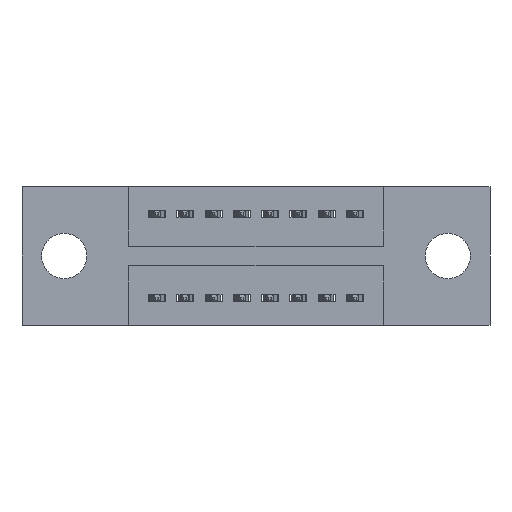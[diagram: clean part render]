
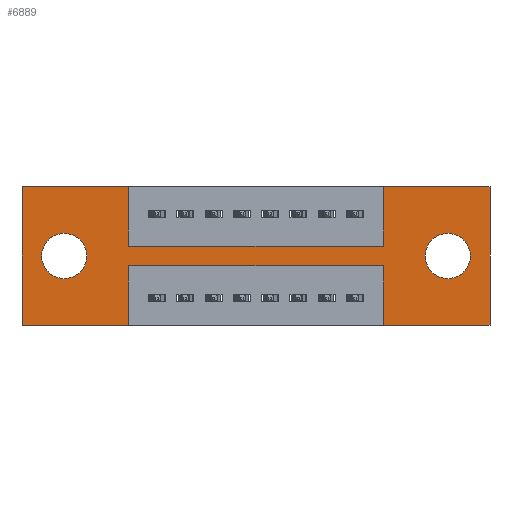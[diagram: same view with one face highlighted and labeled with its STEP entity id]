
A CAD part, front view. The second image highlights one B-rep face of the part: STEP entity #6889.
In plain terms, the highlighted planar face has unit normal (0, -1, 0).
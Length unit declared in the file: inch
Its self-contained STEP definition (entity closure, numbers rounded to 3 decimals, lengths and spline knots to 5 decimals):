
#57 = VECTOR ( 'NONE', #4456, 39.37008 ) ;
#66 = EDGE_CURVE ( 'NONE', #500, #128, #4153, .T. ) ;
#128 = VERTEX_POINT ( 'NONE', #3315 ) ;
#203 = CARTESIAN_POINT ( 'NONE',  ( 0., 0., -0.49 ) ) ;
#219 = VECTOR ( 'NONE', #5042, 39.37008 ) ;
#227 = VECTOR ( 'NONE', #1091, 39.37008 ) ;
#437 = LINE ( 'NONE', #769, #8108 ) ;
#448 = CARTESIAN_POINT ( 'NONE',  ( 1.2775, 0., -0.28 ) ) ;
#485 = CARTESIAN_POINT ( 'NONE',  ( 1.2775, 0., -0.49 ) ) ;
#496 = CARTESIAN_POINT ( 'NONE',  ( 1.5055, 0., -0.245 ) ) ;
#500 = VERTEX_POINT ( 'NONE', #2821 ) ;
#542 = EDGE_CURVE ( 'NONE', #3129, #8382, #5631, .T. ) ;
#664 = CARTESIAN_POINT ( 'NONE',  ( 0.3775, 0., 0. ) ) ;
#678 = VECTOR ( 'NONE', #2033, 39.37008 ) ;
#740 = ORIENTED_EDGE ( 'NONE', *, *, #2849, .T. ) ;
#745 = CARTESIAN_POINT ( 'NONE',  ( 1.655, 0., 0. ) ) ;
#757 = ORIENTED_EDGE ( 'NONE', *, *, #9488, .F. ) ;
#769 = CARTESIAN_POINT ( 'NONE',  ( 0., 0., 0. ) ) ;
#870 = EDGE_LOOP ( 'NONE', ( #5822, #6500 ) ) ;
#881 = VECTOR ( 'NONE', #8742, 39.37008 ) ;
#1036 = CARTESIAN_POINT ( 'NONE',  ( 0.1495, 0., -0.245 ) ) ;
#1091 = DIRECTION ( 'NONE',  ( 1., 0., 0. ) ) ;
#1096 = CARTESIAN_POINT ( 'NONE',  ( 1.2775, 0., -0.28 ) ) ;
#1127 = VECTOR ( 'NONE', #4061, 39.37008 ) ;
#1251 = EDGE_CURVE ( 'NONE', #8382, #4058, #5729, .T. ) ;
#1260 = LINE ( 'NONE', #2525, #227 ) ;
#1397 = ORIENTED_EDGE ( 'NONE', *, *, #8505, .F. ) ;
#1502 = VERTEX_POINT ( 'NONE', #8817 ) ;
#1523 = CARTESIAN_POINT ( 'NONE',  ( 0., 0., -0.49 ) ) ;
#1648 = ORIENTED_EDGE ( 'NONE', *, *, #8785, .F. ) ;
#1735 = VERTEX_POINT ( 'NONE', #3208 ) ;
#1744 = ORIENTED_EDGE ( 'NONE', *, *, #1251, .F. ) ;
#1838 = CARTESIAN_POINT ( 'NONE',  ( 0.3775, 0., -0.49 ) ) ;
#1852 = DIRECTION ( 'NONE',  ( 0., 0., 1. ) ) ;
#1980 = VECTOR ( 'NONE', #4632, 39.37008 ) ;
#2033 = DIRECTION ( 'NONE',  ( 0., 0., 1. ) ) ;
#2076 = LINE ( 'NONE', #5325, #3804 ) ;
#2182 = CARTESIAN_POINT ( 'NONE',  ( 0.3775, 0., -0.21 ) ) ;
#2298 = LINE ( 'NONE', #6245, #1127 ) ;
#2302 = CARTESIAN_POINT ( 'NONE',  ( 0., 0., -0.49 ) ) ;
#2315 = AXIS2_PLACEMENT_3D ( 'NONE', #7726, #9189, #2550 ) ;
#2334 = VERTEX_POINT ( 'NONE', #1838 ) ;
#2390 = EDGE_CURVE ( 'NONE', #1502, #5826, #9069, .T. ) ;
#2414 = EDGE_CURVE ( 'NONE', #128, #500, #7572, .T. ) ;
#2442 = DIRECTION ( 'NONE',  ( 0., -1., 0. ) ) ;
#2525 = CARTESIAN_POINT ( 'NONE',  ( 0., 0., 0. ) ) ;
#2550 = DIRECTION ( 'NONE',  ( 0., 0., 1. ) ) ;
#2821 = CARTESIAN_POINT ( 'NONE',  ( 1.5055, 0., -0.325 ) ) ;
#2849 = EDGE_CURVE ( 'NONE', #5826, #1502, #5921, .T. ) ;
#2871 = LINE ( 'NONE', #2182, #881 ) ;
#2942 = CARTESIAN_POINT ( 'NONE',  ( 0.1495, 0., -0.325 ) ) ;
#3085 = CARTESIAN_POINT ( 'NONE',  ( 0., 0., -0.49 ) ) ;
#3129 = VERTEX_POINT ( 'NONE', #8504 ) ;
#3208 = CARTESIAN_POINT ( 'NONE',  ( 0.3775, 0., -0.21 ) ) ;
#3315 = CARTESIAN_POINT ( 'NONE',  ( 1.5055, 0., -0.165 ) ) ;
#3380 = DIRECTION ( 'NONE',  ( 0., 1., 0. ) ) ;
#3526 = DIRECTION ( 'NONE',  ( 0., 1., 0. ) ) ;
#3633 = ORIENTED_EDGE ( 'NONE', *, *, #8699, .F. ) ;
#3640 = FACE_OUTER_BOUND ( 'NONE', #7630, .T. ) ;
#3703 = VERTEX_POINT ( 'NONE', #745 ) ;
#3729 = DIRECTION ( 'NONE',  ( 0., 0., 1. ) ) ;
#3752 = FACE_BOUND ( 'NONE', #9371, .T. ) ;
#3804 = VECTOR ( 'NONE', #5356, 39.37008 ) ;
#3843 = CARTESIAN_POINT ( 'NONE',  ( 1.5055, 0., -0.245 ) ) ;
#3879 = VECTOR ( 'NONE', #4340, 39.37008 ) ;
#4015 = PLANE ( 'NONE',  #5319 ) ;
#4058 = VERTEX_POINT ( 'NONE', #448 ) ;
#4061 = DIRECTION ( 'NONE',  ( 0., 0., -1. ) ) ;
#4153 = CIRCLE ( 'NONE', #4656, 0.08 ) ;
#4340 = DIRECTION ( 'NONE',  ( 1., 0., 0. ) ) ;
#4456 = DIRECTION ( 'NONE',  ( -1., 0., 0. ) ) ;
#4461 = DIRECTION ( 'NONE',  ( 1., 0., 0. ) ) ;
#4568 = EDGE_CURVE ( 'NONE', #4696, #3703, #437, .T. ) ;
#4632 = DIRECTION ( 'NONE',  ( -1., 0., 0. ) ) ;
#4656 = AXIS2_PLACEMENT_3D ( 'NONE', #3843, #8993, #5355 ) ;
#4696 = VERTEX_POINT ( 'NONE', #5439 ) ;
#4904 = ORIENTED_EDGE ( 'NONE', *, *, #2390, .T. ) ;
#4969 = EDGE_CURVE ( 'NONE', #3703, #3129, #2076, .T. ) ;
#4974 = ORIENTED_EDGE ( 'NONE', *, *, #5094, .F. ) ;
#5042 = DIRECTION ( 'NONE',  ( -1., 0., 0. ) ) ;
#5094 = EDGE_CURVE ( 'NONE', #5318, #1735, #2871, .T. ) ;
#5192 = ORIENTED_EDGE ( 'NONE', *, *, #4969, .F. ) ;
#5318 = VERTEX_POINT ( 'NONE', #664 ) ;
#5319 = AXIS2_PLACEMENT_3D ( 'NONE', #203, #2442, #9113 ) ;
#5325 = CARTESIAN_POINT ( 'NONE',  ( 1.655, 0., 0. ) ) ;
#5355 = DIRECTION ( 'NONE',  ( 0., 0., -1. ) ) ;
#5356 = DIRECTION ( 'NONE',  ( 0., 0., -1. ) ) ;
#5439 = CARTESIAN_POINT ( 'NONE',  ( 1.2775, 0., 0. ) ) ;
#5549 = VERTEX_POINT ( 'NONE', #6957 ) ;
#5631 = LINE ( 'NONE', #1523, #57 ) ;
#5729 = LINE ( 'NONE', #1096, #5839 ) ;
#5822 = ORIENTED_EDGE ( 'NONE', *, *, #2414, .T. ) ;
#5826 = VERTEX_POINT ( 'NONE', #2942 ) ;
#5839 = VECTOR ( 'NONE', #1852, 39.37008 ) ;
#5921 = CIRCLE ( 'NONE', #8960, 0.08 ) ;
#6028 = LINE ( 'NONE', #3085, #1980 ) ;
#6245 = CARTESIAN_POINT ( 'NONE',  ( 0.3775, 0., -0.28 ) ) ;
#6272 = LINE ( 'NONE', #8792, #7438 ) ;
#6305 = CARTESIAN_POINT ( 'NONE',  ( 1.2775, 0., -0.21 ) ) ;
#6435 = CARTESIAN_POINT ( 'NONE',  ( 0.3775, 0., -0.21 ) ) ;
#6500 = ORIENTED_EDGE ( 'NONE', *, *, #66, .T. ) ;
#6549 = EDGE_CURVE ( 'NONE', #1735, #5549, #9522, .T. ) ;
#6630 = VERTEX_POINT ( 'NONE', #8121 ) ;
#6802 = ORIENTED_EDGE ( 'NONE', *, *, #8402, .F. ) ;
#6889 = ADVANCED_FACE ( 'NONE', ( #9514, #3752, #3640 ), #4015, .T. ) ;
#6957 = CARTESIAN_POINT ( 'NONE',  ( 1.2775, 0., -0.21 ) ) ;
#7049 = ORIENTED_EDGE ( 'NONE', *, *, #542, .F. ) ;
#7126 = AXIS2_PLACEMENT_3D ( 'NONE', #496, #3526, #8715 ) ;
#7425 = LINE ( 'NONE', #9466, #219 ) ;
#7438 = VECTOR ( 'NONE', #3729, 39.37008 ) ;
#7532 = ORIENTED_EDGE ( 'NONE', *, *, #4568, .F. ) ;
#7572 = CIRCLE ( 'NONE', #7126, 0.08 ) ;
#7630 = EDGE_LOOP ( 'NONE', ( #9139, #8214, #4974, #3633, #6802, #1397, #757, #1648, #1744, #7049, #5192, #7532 ) ) ;
#7726 = CARTESIAN_POINT ( 'NONE',  ( 0.1495, 0., -0.245 ) ) ;
#8108 = VECTOR ( 'NONE', #4461, 39.37008 ) ;
#8116 = VERTEX_POINT ( 'NONE', #2302 ) ;
#8121 = CARTESIAN_POINT ( 'NONE',  ( 0., 0., 0. ) ) ;
#8125 = VERTEX_POINT ( 'NONE', #8247 ) ;
#8214 = ORIENTED_EDGE ( 'NONE', *, *, #6549, .F. ) ;
#8247 = CARTESIAN_POINT ( 'NONE',  ( 0.3775, 0., -0.28 ) ) ;
#8369 = LINE ( 'NONE', #6305, #678 ) ;
#8382 = VERTEX_POINT ( 'NONE', #485 ) ;
#8402 = EDGE_CURVE ( 'NONE', #8116, #6630, #6272, .T. ) ;
#8494 = DIRECTION ( 'NONE',  ( 0., 0., 1. ) ) ;
#8504 = CARTESIAN_POINT ( 'NONE',  ( 1.655, 0., -0.49 ) ) ;
#8505 = EDGE_CURVE ( 'NONE', #2334, #8116, #6028, .T. ) ;
#8699 = EDGE_CURVE ( 'NONE', #6630, #5318, #1260, .T. ) ;
#8715 = DIRECTION ( 'NONE',  ( 0., 0., -1. ) ) ;
#8742 = DIRECTION ( 'NONE',  ( 0., 0., -1. ) ) ;
#8785 = EDGE_CURVE ( 'NONE', #4058, #8125, #7425, .T. ) ;
#8792 = CARTESIAN_POINT ( 'NONE',  ( 0., 0., 0. ) ) ;
#8817 = CARTESIAN_POINT ( 'NONE',  ( 0.1495, 0., -0.165 ) ) ;
#8876 = EDGE_CURVE ( 'NONE', #5549, #4696, #8369, .T. ) ;
#8960 = AXIS2_PLACEMENT_3D ( 'NONE', #1036, #3380, #8494 ) ;
#8993 = DIRECTION ( 'NONE',  ( 0., 1., 0. ) ) ;
#9069 = CIRCLE ( 'NONE', #2315, 0.08 ) ;
#9113 = DIRECTION ( 'NONE',  ( 0., 0., -1. ) ) ;
#9139 = ORIENTED_EDGE ( 'NONE', *, *, #8876, .F. ) ;
#9189 = DIRECTION ( 'NONE',  ( 0., 1., 0. ) ) ;
#9371 = EDGE_LOOP ( 'NONE', ( #4904, #740 ) ) ;
#9466 = CARTESIAN_POINT ( 'NONE',  ( 0.3775, 0., -0.28 ) ) ;
#9488 = EDGE_CURVE ( 'NONE', #8125, #2334, #2298, .T. ) ;
#9514 = FACE_BOUND ( 'NONE', #870, .T. ) ;
#9522 = LINE ( 'NONE', #6435, #3879 ) ;
